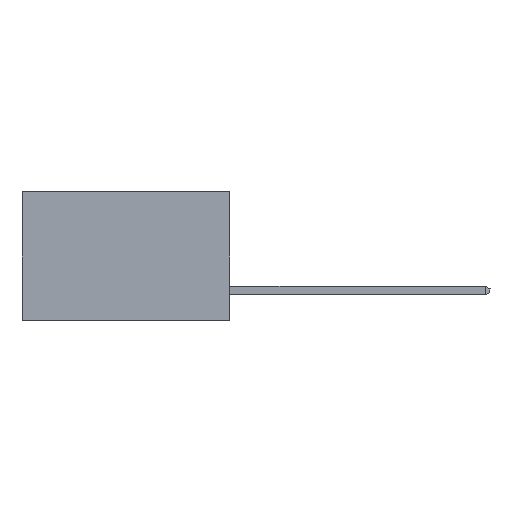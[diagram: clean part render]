
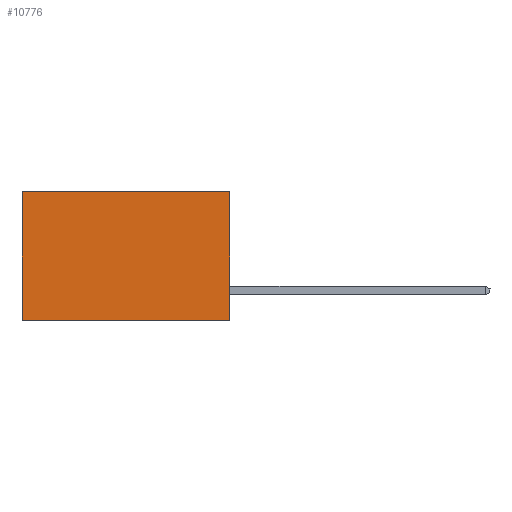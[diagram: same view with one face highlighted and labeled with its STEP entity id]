
A CAD part, left-side view. The second image highlights one B-rep face of the part: STEP entity #10776.
In plain terms, the highlighted planar face has unit normal (-1, 0, 0).
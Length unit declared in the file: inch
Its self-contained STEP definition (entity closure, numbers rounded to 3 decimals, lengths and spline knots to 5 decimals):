
#938 = LINE ( 'NONE', #17968, #15359 ) ;
#1638 = VERTEX_POINT ( 'NONE', #15650 ) ;
#1941 = CARTESIAN_POINT ( 'NONE',  ( 0.2615, 0.6, -0.37 ) ) ;
#2314 = EDGE_CURVE ( 'NONE', #1638, #11896, #938, .T. ) ;
#2440 = DIRECTION ( 'NONE',  ( 0., 1., 0. ) ) ;
#3058 = CARTESIAN_POINT ( 'NONE',  ( 0.2615, 0., -0.37 ) ) ;
#3227 = DIRECTION ( 'NONE',  ( 1., 0., 0. ) ) ;
#4121 = ORIENTED_EDGE ( 'NONE', *, *, #15710, .T. ) ;
#4261 = CARTESIAN_POINT ( 'NONE',  ( 0.2615, 0., -0.37 ) ) ;
#5321 = LINE ( 'NONE', #13733, #17387 ) ;
#6633 = EDGE_LOOP ( 'NONE', ( #4121, #11808, #13186, #11314 ) ) ;
#7387 = DIRECTION ( 'NONE',  ( 0., 0., -1. ) ) ;
#8030 = DIRECTION ( 'NONE',  ( 0., 0., -1. ) ) ;
#8118 = VERTEX_POINT ( 'NONE', #1941 ) ;
#8646 = DIRECTION ( 'NONE',  ( 0., 1., 0. ) ) ;
#8853 = CARTESIAN_POINT ( 'NONE',  ( 0.2615, 0.6, 0. ) ) ;
#9118 = FACE_OUTER_BOUND ( 'NONE', #6633, .T. ) ;
#9624 = LINE ( 'NONE', #4261, #11876 ) ;
#10098 = CARTESIAN_POINT ( 'NONE',  ( 0.2615, 0., 0. ) ) ;
#10776 = ADVANCED_FACE ( 'NONE', ( #9118 ), #14688, .F. ) ;
#11314 = ORIENTED_EDGE ( 'NONE', *, *, #17462, .T. ) ;
#11478 = LINE ( 'NONE', #10098, #13369 ) ;
#11808 = ORIENTED_EDGE ( 'NONE', *, *, #15350, .F. ) ;
#11876 = VECTOR ( 'NONE', #2440, 39.37008 ) ;
#11896 = VERTEX_POINT ( 'NONE', #3058 ) ;
#12552 = VERTEX_POINT ( 'NONE', #8853 ) ;
#13186 = ORIENTED_EDGE ( 'NONE', *, *, #2314, .F. ) ;
#13369 = VECTOR ( 'NONE', #8646, 39.37008 ) ;
#13733 = CARTESIAN_POINT ( 'NONE',  ( 0.2615, 0.6, -0.37 ) ) ;
#14105 = AXIS2_PLACEMENT_3D ( 'NONE', #15692, #3227, #7387 ) ;
#14688 = PLANE ( 'NONE',  #14105 ) ;
#15350 = EDGE_CURVE ( 'NONE', #11896, #8118, #9624, .T. ) ;
#15359 = VECTOR ( 'NONE', #8030, 39.37008 ) ;
#15650 = CARTESIAN_POINT ( 'NONE',  ( 0.2615, 0., 0. ) ) ;
#15692 = CARTESIAN_POINT ( 'NONE',  ( 0.2615, 0., -0.37 ) ) ;
#15710 = EDGE_CURVE ( 'NONE', #12552, #8118, #5321, .T. ) ;
#16617 = DIRECTION ( 'NONE',  ( 0., 0., -1. ) ) ;
#17387 = VECTOR ( 'NONE', #16617, 39.37008 ) ;
#17462 = EDGE_CURVE ( 'NONE', #1638, #12552, #11478, .T. ) ;
#17968 = CARTESIAN_POINT ( 'NONE',  ( 0.2615, 0., -0.37 ) ) ;
